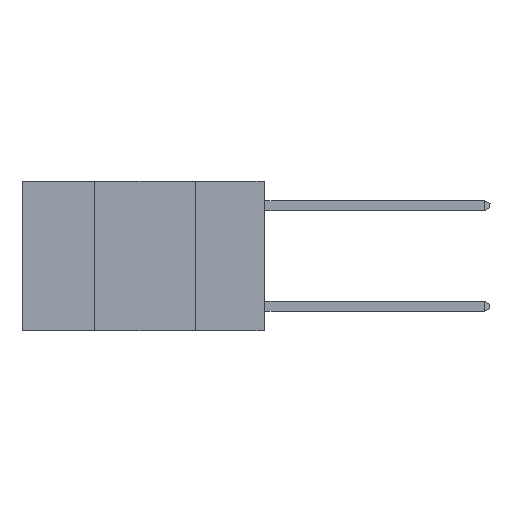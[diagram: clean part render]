
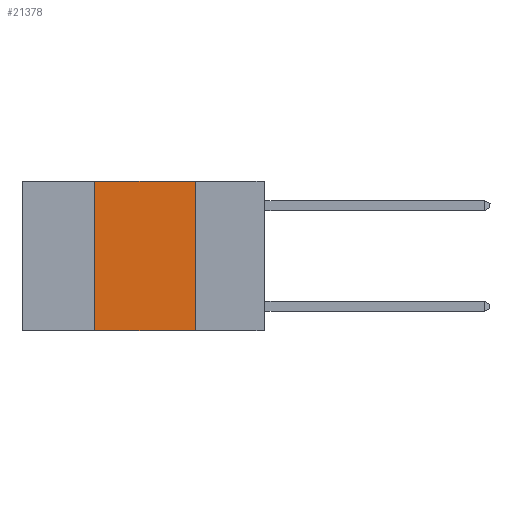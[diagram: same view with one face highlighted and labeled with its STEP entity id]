
A CAD part, left-side view. The second image highlights one B-rep face of the part: STEP entity #21378.
In plain terms, the highlighted planar face has unit normal (-1, 0, 0).
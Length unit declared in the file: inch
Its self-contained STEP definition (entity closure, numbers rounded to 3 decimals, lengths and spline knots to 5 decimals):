
#100 = CARTESIAN_POINT ( 'NONE',  ( 0., 0.42, 0. ) ) ;
#405 = EDGE_CURVE ( 'NONE', #4680, #2916, #21164, .T. ) ;
#1790 = DIRECTION ( 'NONE',  ( 1., 0., 0. ) ) ;
#2916 = VERTEX_POINT ( 'NONE', #100 ) ;
#4217 = EDGE_LOOP ( 'NONE', ( #7411, #28104, #28457, #20890 ) ) ;
#4649 = LINE ( 'NONE', #27594, #16374 ) ;
#4680 = VERTEX_POINT ( 'NONE', #20894 ) ;
#6572 = VERTEX_POINT ( 'NONE', #6579 ) ;
#6579 = CARTESIAN_POINT ( 'NONE',  ( 0., 0.17, -0.37 ) ) ;
#7411 = ORIENTED_EDGE ( 'NONE', *, *, #8528, .F. ) ;
#8528 = EDGE_CURVE ( 'NONE', #29335, #6572, #8933, .T. ) ;
#8933 = LINE ( 'NONE', #27837, #13906 ) ;
#9055 = DIRECTION ( 'NONE',  ( 0., -1., 0. ) ) ;
#11085 = DIRECTION ( 'NONE',  ( 0., 0., -1. ) ) ;
#13117 = FACE_OUTER_BOUND ( 'NONE', #4217, .T. ) ;
#13906 = VECTOR ( 'NONE', #22738, 39.37008 ) ;
#14902 = AXIS2_PLACEMENT_3D ( 'NONE', #24907, #1790, #11085 ) ;
#16208 = CARTESIAN_POINT ( 'NONE',  ( 0., 0.42, 0. ) ) ;
#16374 = VECTOR ( 'NONE', #25746, 39.37008 ) ;
#16768 = VECTOR ( 'NONE', #21326, 39.37008 ) ;
#18978 = LINE ( 'NONE', #23619, #24009 ) ;
#20023 = CARTESIAN_POINT ( 'NONE',  ( 0., 0.17, 0. ) ) ;
#20890 = ORIENTED_EDGE ( 'NONE', *, *, #21024, .T. ) ;
#20894 = CARTESIAN_POINT ( 'NONE',  ( 0., 0.42, -0.37 ) ) ;
#21024 = EDGE_CURVE ( 'NONE', #4680, #6572, #4649, .T. ) ;
#21164 = LINE ( 'NONE', #16208, #16768 ) ;
#21326 = DIRECTION ( 'NONE',  ( 0., 0., 1. ) ) ;
#21378 = ADVANCED_FACE ( 'NONE', ( #13117 ), #27830, .F. ) ;
#22738 = DIRECTION ( 'NONE',  ( 0., 0., -1. ) ) ;
#23619 = CARTESIAN_POINT ( 'NONE',  ( 0., 0.6, 0. ) ) ;
#24009 = VECTOR ( 'NONE', #9055, 39.37008 ) ;
#24907 = CARTESIAN_POINT ( 'NONE',  ( 0., 0.6, 0. ) ) ;
#25746 = DIRECTION ( 'NONE',  ( 0., -1., 0. ) ) ;
#27594 = CARTESIAN_POINT ( 'NONE',  ( 0., 0.6, -0.37 ) ) ;
#27830 = PLANE ( 'NONE',  #14902 ) ;
#27837 = CARTESIAN_POINT ( 'NONE',  ( 0., 0.17, 0. ) ) ;
#27937 = EDGE_CURVE ( 'NONE', #2916, #29335, #18978, .T. ) ;
#28104 = ORIENTED_EDGE ( 'NONE', *, *, #27937, .F. ) ;
#28457 = ORIENTED_EDGE ( 'NONE', *, *, #405, .F. ) ;
#29335 = VERTEX_POINT ( 'NONE', #20023 ) ;
